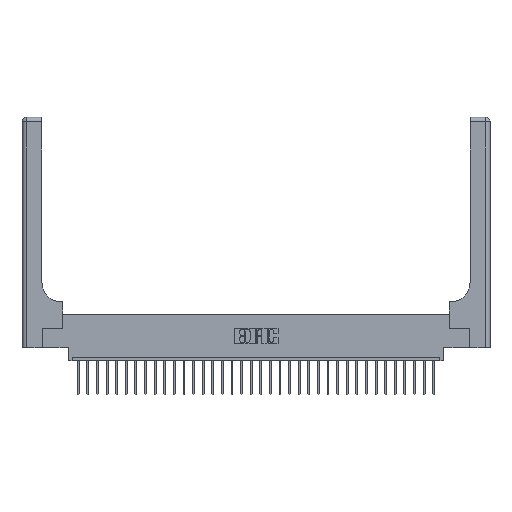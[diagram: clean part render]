
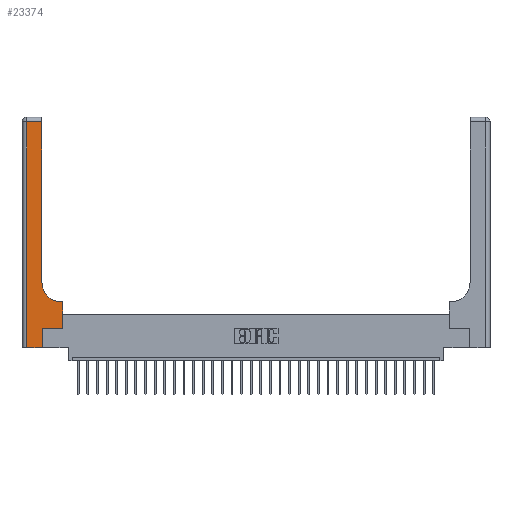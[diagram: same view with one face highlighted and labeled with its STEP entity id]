
A CAD part, top view. The second image highlights one B-rep face of the part: STEP entity #23374.
In plain terms, the highlighted planar face has unit normal (0, 0, 1).
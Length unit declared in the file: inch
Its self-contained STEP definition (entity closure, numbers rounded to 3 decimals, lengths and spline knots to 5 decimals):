
#53 = VECTOR ( 'NONE', #13192, 39.37008 ) ;
#536 = ORIENTED_EDGE ( 'NONE', *, *, #11408, .T. ) ;
#638 = DIRECTION ( 'NONE',  ( 0., 0., -1. ) ) ;
#690 = VERTEX_POINT ( 'NONE', #16057 ) ;
#1063 = EDGE_CURVE ( 'NONE', #5762, #4018, #18518, .T. ) ;
#1123 = VERTEX_POINT ( 'NONE', #27915 ) ;
#2009 = ORIENTED_EDGE ( 'NONE', *, *, #1063, .T. ) ;
#2963 = DIRECTION ( 'NONE',  ( 0., 1., 0. ) ) ;
#3151 = LINE ( 'NONE', #20518, #14527 ) ;
#3260 = LINE ( 'NONE', #10825, #53 ) ;
#3310 = LINE ( 'NONE', #21633, #17574 ) ;
#3399 = CARTESIAN_POINT ( 'NONE',  ( 0.265, 0., 0.37 ) ) ;
#3431 = VERTEX_POINT ( 'NONE', #7021 ) ;
#3762 = EDGE_CURVE ( 'NONE', #4617, #8964, #26907, .T. ) ;
#4018 = VERTEX_POINT ( 'NONE', #9563 ) ;
#4278 = ORIENTED_EDGE ( 'NONE', *, *, #23937, .T. ) ;
#4617 = VERTEX_POINT ( 'NONE', #16807 ) ;
#4976 = DIRECTION ( 'NONE',  ( 1., 0., 0. ) ) ;
#5332 = LINE ( 'NONE', #21031, #21392 ) ;
#5762 = VERTEX_POINT ( 'NONE', #24676 ) ;
#7021 = CARTESIAN_POINT ( 'NONE',  ( 0.265, 0.25, 0.37 ) ) ;
#7238 = CARTESIAN_POINT ( 'NONE',  ( 0.06, 3., 0.37 ) ) ;
#8964 = VERTEX_POINT ( 'NONE', #29169 ) ;
#9128 = CARTESIAN_POINT ( 'NONE',  ( 0.528, 0.25, 0.37 ) ) ;
#9563 = CARTESIAN_POINT ( 'NONE',  ( 0.06, 0., 0.37 ) ) ;
#10194 = EDGE_CURVE ( 'NONE', #1123, #690, #3310, .T. ) ;
#10825 = CARTESIAN_POINT ( 'NONE',  ( 0.265, 0.25, 0.37 ) ) ;
#10860 = EDGE_LOOP ( 'NONE', ( #24404, #20738, #2009, #28455, #22076, #17272, #536, #25643, #4278 ) ) ;
#11408 = EDGE_CURVE ( 'NONE', #25911, #1123, #17492, .T. ) ;
#11903 = AXIS2_PLACEMENT_3D ( 'NONE', #16224, #25331, #4976 ) ;
#13192 = DIRECTION ( 'NONE',  ( 1., 0., 0. ) ) ;
#14527 = VECTOR ( 'NONE', #2963, 39.37008 ) ;
#14749 = DIRECTION ( 'NONE',  ( 0., 1., 0. ) ) ;
#15984 = LINE ( 'NONE', #29216, #17061 ) ;
#16057 = CARTESIAN_POINT ( 'NONE',  ( 0.51, 0.6, 0.37 ) ) ;
#16069 = CARTESIAN_POINT ( 'NONE',  ( 0.26, 3., 0.37 ) ) ;
#16224 = CARTESIAN_POINT ( 'NONE',  ( 0.51, 0.85, 0.37 ) ) ;
#16587 = DIRECTION ( 'NONE',  ( 0., -1., 0. ) ) ;
#16807 = CARTESIAN_POINT ( 'NONE',  ( 0.26, 0.85, 0.37 ) ) ;
#16843 = DIRECTION ( 'NONE',  ( -1., 0., 0. ) ) ;
#17061 = VECTOR ( 'NONE', #19813, 39.37008 ) ;
#17272 = ORIENTED_EDGE ( 'NONE', *, *, #21137, .T. ) ;
#17492 = LINE ( 'NONE', #20226, #21773 ) ;
#17574 = VECTOR ( 'NONE', #16843, 39.37008 ) ;
#18110 = FACE_OUTER_BOUND ( 'NONE', #10860, .T. ) ;
#18237 = AXIS2_PLACEMENT_3D ( 'NONE', #23444, #638, #25835 ) ;
#18518 = LINE ( 'NONE', #7238, #28098 ) ;
#19117 = CIRCLE ( 'NONE', #11903, 0.25 ) ;
#19813 = DIRECTION ( 'NONE',  ( 1., 0., 0. ) ) ;
#20226 = CARTESIAN_POINT ( 'NONE',  ( 0.528, 0.25, 0.37 ) ) ;
#20469 = VERTEX_POINT ( 'NONE', #3399 ) ;
#20518 = CARTESIAN_POINT ( 'NONE',  ( 0.265, 0., 0.37 ) ) ;
#20738 = ORIENTED_EDGE ( 'NONE', *, *, #21790, .T. ) ;
#20848 = VECTOR ( 'NONE', #14749, 39.37008 ) ;
#21031 = CARTESIAN_POINT ( 'NONE',  ( 0., 2.94, 0.37 ) ) ;
#21137 = EDGE_CURVE ( 'NONE', #3431, #25911, #3260, .T. ) ;
#21392 = VECTOR ( 'NONE', #25645, 39.37008 ) ;
#21633 = CARTESIAN_POINT ( 'NONE',  ( 0.26, 0.6, 0.37 ) ) ;
#21773 = VECTOR ( 'NONE', #22631, 39.37008 ) ;
#21790 = EDGE_CURVE ( 'NONE', #8964, #5762, #5332, .T. ) ;
#22076 = ORIENTED_EDGE ( 'NONE', *, *, #27420, .T. ) ;
#22631 = DIRECTION ( 'NONE',  ( 0., 1., 0. ) ) ;
#22658 = EDGE_CURVE ( 'NONE', #4018, #20469, #15984, .T. ) ;
#23342 = PLANE ( 'NONE',  #18237 ) ;
#23374 = ADVANCED_FACE ( 'NONE', ( #18110 ), #23342, .F. ) ;
#23444 = CARTESIAN_POINT ( 'NONE',  ( 0., 3., 0.37 ) ) ;
#23937 = EDGE_CURVE ( 'NONE', #690, #4617, #19117, .T. ) ;
#24404 = ORIENTED_EDGE ( 'NONE', *, *, #3762, .T. ) ;
#24676 = CARTESIAN_POINT ( 'NONE',  ( 0.06, 2.94, 0.37 ) ) ;
#25331 = DIRECTION ( 'NONE',  ( 0., 0., -1. ) ) ;
#25643 = ORIENTED_EDGE ( 'NONE', *, *, #10194, .T. ) ;
#25645 = DIRECTION ( 'NONE',  ( -1., 0., 0. ) ) ;
#25835 = DIRECTION ( 'NONE',  ( -1., 0., 0. ) ) ;
#25911 = VERTEX_POINT ( 'NONE', #9128 ) ;
#26907 = LINE ( 'NONE', #16069, #20848 ) ;
#27420 = EDGE_CURVE ( 'NONE', #20469, #3431, #3151, .T. ) ;
#27915 = CARTESIAN_POINT ( 'NONE',  ( 0.528, 0.6, 0.37 ) ) ;
#28098 = VECTOR ( 'NONE', #16587, 39.37008 ) ;
#28455 = ORIENTED_EDGE ( 'NONE', *, *, #22658, .T. ) ;
#29169 = CARTESIAN_POINT ( 'NONE',  ( 0.26, 2.94, 0.37 ) ) ;
#29216 = CARTESIAN_POINT ( 'NONE',  ( 0., 0., 0.37 ) ) ;
